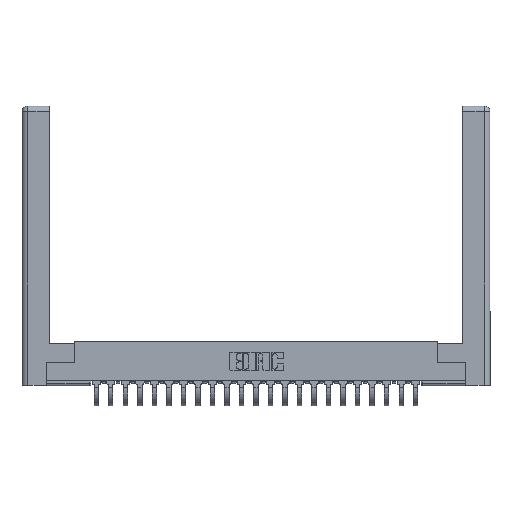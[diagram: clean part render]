
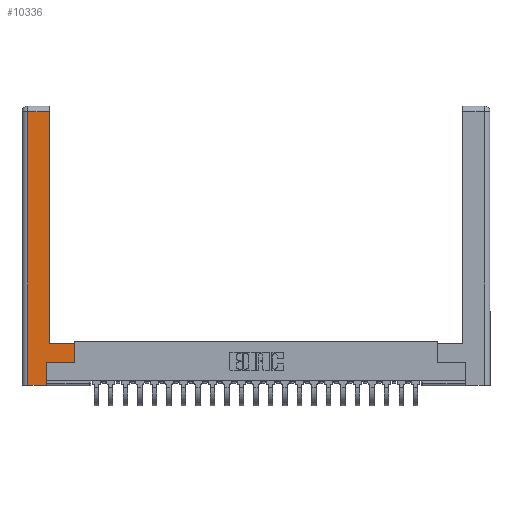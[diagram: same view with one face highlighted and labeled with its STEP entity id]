
A CAD part, top view. The second image highlights one B-rep face of the part: STEP entity #10336.
In plain terms, the highlighted planar face has unit normal (0, 0, 1).
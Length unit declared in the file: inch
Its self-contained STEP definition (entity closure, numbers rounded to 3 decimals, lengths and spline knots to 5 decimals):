
#520 = VERTEX_POINT ( 'NONE', #7294 ) ;
#1112 = PLANE ( 'NONE',  #13541 ) ;
#1255 = ORIENTED_EDGE ( 'NONE', *, *, #21825, .T. ) ;
#1424 = ORIENTED_EDGE ( 'NONE', *, *, #2052, .T. ) ;
#1459 = LINE ( 'NONE', #24345, #16178 ) ;
#1825 = ORIENTED_EDGE ( 'NONE', *, *, #4007, .T. ) ;
#2052 = EDGE_CURVE ( 'NONE', #23832, #15401, #1459, .T. ) ;
#2123 = VECTOR ( 'NONE', #24083, 39.37008 ) ;
#2307 = VECTOR ( 'NONE', #13769, 39.37008 ) ;
#2611 = DIRECTION ( 'NONE',  ( -1., 0., 0. ) ) ;
#3190 = CARTESIAN_POINT ( 'NONE',  ( 0.295, 0.45, 0. ) ) ;
#3258 = CARTESIAN_POINT ( 'NONE',  ( 0.265, 0., 0. ) ) ;
#3455 = CARTESIAN_POINT ( 'NONE',  ( 0.295, 3., 0. ) ) ;
#3788 = ORIENTED_EDGE ( 'NONE', *, *, #12364, .T. ) ;
#4007 = EDGE_CURVE ( 'NONE', #5836, #520, #15800, .T. ) ;
#5160 = CARTESIAN_POINT ( 'NONE',  ( 0.0615, 0., 0. ) ) ;
#5790 = VERTEX_POINT ( 'NONE', #9249 ) ;
#5836 = VERTEX_POINT ( 'NONE', #7730 ) ;
#6961 = EDGE_CURVE ( 'NONE', #9340, #5790, #7829, .T. ) ;
#7246 = LINE ( 'NONE', #25905, #18786 ) ;
#7294 = CARTESIAN_POINT ( 'NONE',  ( 0.265, 0., 0. ) ) ;
#7458 = LINE ( 'NONE', #15763, #2123 ) ;
#7730 = CARTESIAN_POINT ( 'NONE',  ( 0.0615, 0., 0. ) ) ;
#7765 = VERTEX_POINT ( 'NONE', #12375 ) ;
#7829 = LINE ( 'NONE', #3455, #11503 ) ;
#8590 = CARTESIAN_POINT ( 'NONE',  ( 0.295, 0.45, 0. ) ) ;
#9027 = DIRECTION ( 'NONE',  ( -1., 0., 0. ) ) ;
#9249 = CARTESIAN_POINT ( 'NONE',  ( 0.295, 2.94, 0. ) ) ;
#9340 = VERTEX_POINT ( 'NONE', #8590 ) ;
#9595 = DIRECTION ( 'NONE',  ( -1., 0., 0. ) ) ;
#9729 = LINE ( 'NONE', #3190, #23337 ) ;
#10336 = ADVANCED_FACE ( 'NONE', ( #19650 ), #1112, .F. ) ;
#10566 = ORIENTED_EDGE ( 'NONE', *, *, #20407, .T. ) ;
#11503 = VECTOR ( 'NONE', #20250, 39.37008 ) ;
#12076 = CARTESIAN_POINT ( 'NONE',  ( 0.565, 0.245, 0. ) ) ;
#12364 = EDGE_CURVE ( 'NONE', #5790, #17324, #7246, .T. ) ;
#12375 = CARTESIAN_POINT ( 'NONE',  ( 0.265, 0.245, 0. ) ) ;
#13541 = AXIS2_PLACEMENT_3D ( 'NONE', #21439, #15293, #9027 ) ;
#13769 = DIRECTION ( 'NONE',  ( 1., 0., 0. ) ) ;
#14299 = DIRECTION ( 'NONE',  ( 0., 1., 0. ) ) ;
#15293 = DIRECTION ( 'NONE',  ( 0., 0., -1. ) ) ;
#15401 = VERTEX_POINT ( 'NONE', #19344 ) ;
#15763 = CARTESIAN_POINT ( 'NONE',  ( 0.565, 0.245, 0. ) ) ;
#15800 = LINE ( 'NONE', #3258, #2307 ) ;
#16178 = VECTOR ( 'NONE', #22311, 39.37008 ) ;
#16485 = ORIENTED_EDGE ( 'NONE', *, *, #26683, .T. ) ;
#17324 = VERTEX_POINT ( 'NONE', #26497 ) ;
#17733 = EDGE_LOOP ( 'NONE', ( #23866, #3788, #19730, #1825, #16485, #1255, #1424, #10566 ) ) ;
#18786 = VECTOR ( 'NONE', #2611, 39.37008 ) ;
#19344 = CARTESIAN_POINT ( 'NONE',  ( 0.565, 0.45, 0. ) ) ;
#19650 = FACE_OUTER_BOUND ( 'NONE', #17733, .T. ) ;
#19730 = ORIENTED_EDGE ( 'NONE', *, *, #22685, .T. ) ;
#20161 = LINE ( 'NONE', #25189, #24032 ) ;
#20250 = DIRECTION ( 'NONE',  ( 0., 1., 0. ) ) ;
#20407 = EDGE_CURVE ( 'NONE', #15401, #9340, #9729, .T. ) ;
#21439 = CARTESIAN_POINT ( 'NONE',  ( 0., 0., 0. ) ) ;
#21825 = EDGE_CURVE ( 'NONE', #7765, #23832, #7458, .T. ) ;
#22311 = DIRECTION ( 'NONE',  ( 0., 1., 0. ) ) ;
#22556 = VECTOR ( 'NONE', #23847, 39.37008 ) ;
#22685 = EDGE_CURVE ( 'NONE', #17324, #5836, #23723, .T. ) ;
#23337 = VECTOR ( 'NONE', #9595, 39.37008 ) ;
#23723 = LINE ( 'NONE', #5160, #22556 ) ;
#23832 = VERTEX_POINT ( 'NONE', #12076 ) ;
#23847 = DIRECTION ( 'NONE',  ( 0., -1., 0. ) ) ;
#23866 = ORIENTED_EDGE ( 'NONE', *, *, #6961, .T. ) ;
#24032 = VECTOR ( 'NONE', #14299, 39.37008 ) ;
#24083 = DIRECTION ( 'NONE',  ( 1., 0., 0. ) ) ;
#24345 = CARTESIAN_POINT ( 'NONE',  ( 0.565, 0.45, 0. ) ) ;
#25189 = CARTESIAN_POINT ( 'NONE',  ( 0.265, 0.245, 0. ) ) ;
#25905 = CARTESIAN_POINT ( 'NONE',  ( 0.0615, 2.94, 0. ) ) ;
#26497 = CARTESIAN_POINT ( 'NONE',  ( 0.0615, 2.94, 0. ) ) ;
#26683 = EDGE_CURVE ( 'NONE', #520, #7765, #20161, .T. ) ;
